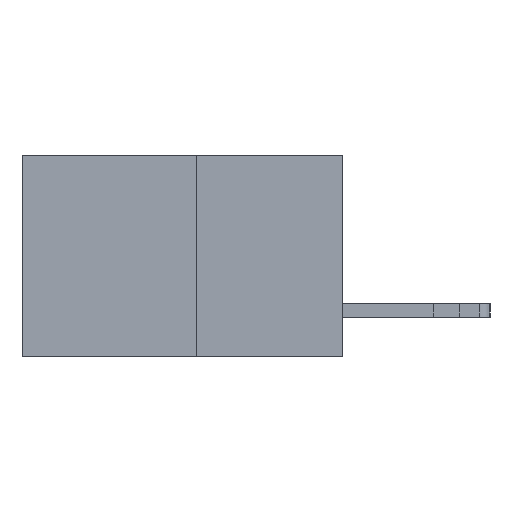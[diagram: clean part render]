
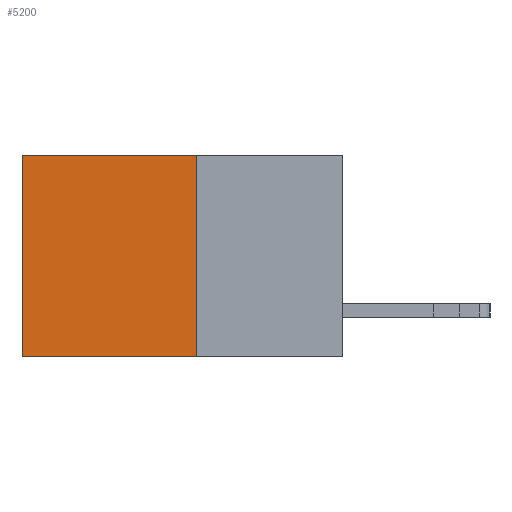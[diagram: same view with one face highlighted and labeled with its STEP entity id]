
A CAD part, left-side view. The second image highlights one B-rep face of the part: STEP entity #5200.
In plain terms, the highlighted planar face has unit normal (-1, 0, 0).
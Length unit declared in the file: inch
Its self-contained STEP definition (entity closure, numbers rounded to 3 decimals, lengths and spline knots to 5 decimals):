
#29 = DIRECTION ( 'NONE',  ( 0., 0., -1. ) ) ;
#268 = VECTOR ( 'NONE', #1719, 39.37008 ) ;
#322 = VERTEX_POINT ( 'NONE', #11849 ) ;
#1719 = DIRECTION ( 'NONE',  ( 0., 1., 0. ) ) ;
#2584 = ORIENTED_EDGE ( 'NONE', *, *, #18988, .T. ) ;
#2780 = PLANE ( 'NONE',  #16183 ) ;
#3546 = CARTESIAN_POINT ( 'NONE',  ( 0.277, 0.59, -0.37 ) ) ;
#4040 = VERTEX_POINT ( 'NONE', #9712 ) ;
#4897 = ORIENTED_EDGE ( 'NONE', *, *, #5677, .F. ) ;
#5200 = ADVANCED_FACE ( 'NONE', ( #20093 ), #2780, .F. ) ;
#5677 = EDGE_CURVE ( 'NONE', #8824, #12211, #18452, .T. ) ;
#6205 = DIRECTION ( 'NONE',  ( 1., 0., 0. ) ) ;
#8648 = ORIENTED_EDGE ( 'NONE', *, *, #22260, .F. ) ;
#8815 = CARTESIAN_POINT ( 'NONE',  ( 0.277, 0.27, -0.37 ) ) ;
#8824 = VERTEX_POINT ( 'NONE', #12444 ) ;
#8899 = VECTOR ( 'NONE', #29, 39.37008 ) ;
#9446 = LINE ( 'NONE', #12017, #268 ) ;
#9712 = CARTESIAN_POINT ( 'NONE',  ( 0.277, 0.27, 0. ) ) ;
#9835 = VECTOR ( 'NONE', #12571, 39.37008 ) ;
#10533 = DIRECTION ( 'NONE',  ( 0., 0., -1. ) ) ;
#10848 = CARTESIAN_POINT ( 'NONE',  ( 0.277, 0.27, -0.37 ) ) ;
#11205 = ORIENTED_EDGE ( 'NONE', *, *, #18968, .T. ) ;
#11849 = CARTESIAN_POINT ( 'NONE',  ( 0.277, 0.59, 0. ) ) ;
#12017 = CARTESIAN_POINT ( 'NONE',  ( 0.277, 0.27, 0. ) ) ;
#12053 = LINE ( 'NONE', #8815, #20682 ) ;
#12211 = VERTEX_POINT ( 'NONE', #3546 ) ;
#12444 = CARTESIAN_POINT ( 'NONE',  ( 0.277, 0.27, -0.37 ) ) ;
#12571 = DIRECTION ( 'NONE',  ( 0., 1., 0. ) ) ;
#16155 = EDGE_LOOP ( 'NONE', ( #2584, #4897, #8648, #11205 ) ) ;
#16183 = AXIS2_PLACEMENT_3D ( 'NONE', #18173, #6205, #18241 ) ;
#18054 = LINE ( 'NONE', #20538, #8899 ) ;
#18173 = CARTESIAN_POINT ( 'NONE',  ( 0.277, 0.27, -0.37 ) ) ;
#18241 = DIRECTION ( 'NONE',  ( 0., 0., -1. ) ) ;
#18452 = LINE ( 'NONE', #10848, #9835 ) ;
#18968 = EDGE_CURVE ( 'NONE', #4040, #322, #9446, .T. ) ;
#18988 = EDGE_CURVE ( 'NONE', #322, #12211, #18054, .T. ) ;
#20093 = FACE_OUTER_BOUND ( 'NONE', #16155, .T. ) ;
#20538 = CARTESIAN_POINT ( 'NONE',  ( 0.277, 0.59, -0.37 ) ) ;
#20682 = VECTOR ( 'NONE', #10533, 39.37008 ) ;
#22260 = EDGE_CURVE ( 'NONE', #4040, #8824, #12053, .T. ) ;
